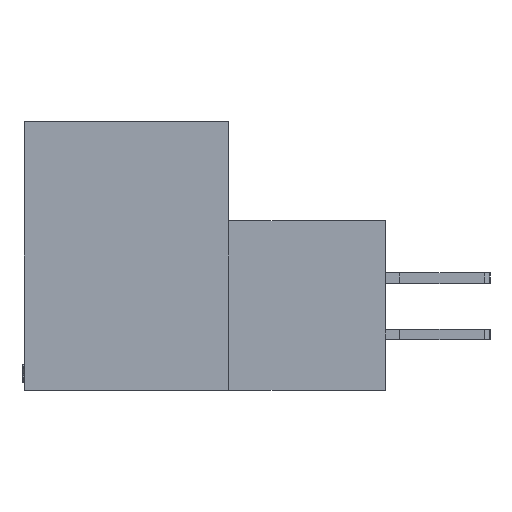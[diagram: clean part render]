
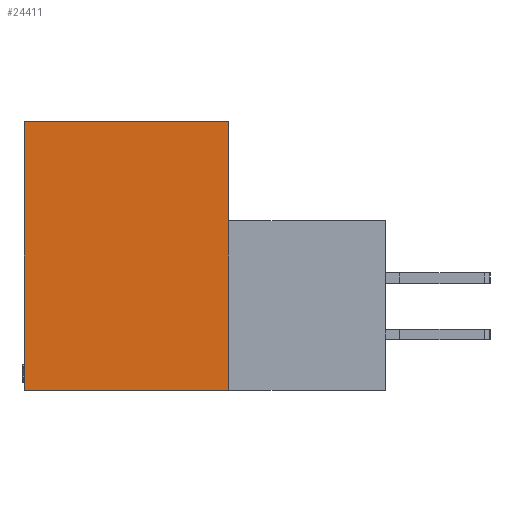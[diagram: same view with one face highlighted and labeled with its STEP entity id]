
A CAD part, left-side view. The second image highlights one B-rep face of the part: STEP entity #24411.
In plain terms, the highlighted planar face has unit normal (-1, 0, 0).
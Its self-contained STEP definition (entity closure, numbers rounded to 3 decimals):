
#324 = EDGE_LOOP ( 'NONE', ( #28597, #47243, #20728, #26605 ) ) ;
#6104 = VERTEX_POINT ( 'NONE', #22603 ) ;
#8108 = DIRECTION ( 'NONE',  ( 0., 1., 0. ) ) ;
#8125 = CARTESIAN_POINT ( 'NONE',  ( 0., 11.506, 0. ) ) ;
#10813 = CARTESIAN_POINT ( 'NONE',  ( 0., 11.506, 0. ) ) ;
#12342 = VERTEX_POINT ( 'NONE', #8125 ) ;
#13488 = DIRECTION ( 'NONE',  ( 0., 0., 1. ) ) ;
#13657 = EDGE_CURVE ( 'NONE', #35111, #43750, #15766, .T. ) ;
#13810 = VECTOR ( 'NONE', #13488, 1000. ) ;
#14408 = EDGE_CURVE ( 'NONE', #43750, #12342, #45364, .T. ) ;
#15766 = LINE ( 'NONE', #31587, #33602 ) ;
#15877 = VECTOR ( 'NONE', #19245, 1000. ) ;
#18761 = PLANE ( 'NONE',  #49935 ) ;
#18810 = CARTESIAN_POINT ( 'NONE',  ( 0., 11.506, -15.088 ) ) ;
#18910 = CARTESIAN_POINT ( 'NONE',  ( 0., 0., 0. ) ) ;
#18948 = CARTESIAN_POINT ( 'NONE',  ( 0., 0., 0. ) ) ;
#19245 = DIRECTION ( 'NONE',  ( 0., 0., -1. ) ) ;
#20728 = ORIENTED_EDGE ( 'NONE', *, *, #32655, .F. ) ;
#22603 = CARTESIAN_POINT ( 'NONE',  ( 0., 0., 0. ) ) ;
#24107 = LINE ( 'NONE', #10813, #32797 ) ;
#24411 = ADVANCED_FACE ( 'NONE', ( #40048 ), #18761, .F. ) ;
#26605 = ORIENTED_EDGE ( 'NONE', *, *, #14408, .F. ) ;
#26664 = DIRECTION ( 'NONE',  ( 0., 0., -1. ) ) ;
#28597 = ORIENTED_EDGE ( 'NONE', *, *, #13657, .F. ) ;
#31587 = CARTESIAN_POINT ( 'NONE',  ( 0., -8.814, -15.088 ) ) ;
#32655 = EDGE_CURVE ( 'NONE', #12342, #6104, #24107, .T. ) ;
#32797 = VECTOR ( 'NONE', #34299, 1000. ) ;
#33602 = VECTOR ( 'NONE', #8108, 1000. ) ;
#34299 = DIRECTION ( 'NONE',  ( 0., -1., 0. ) ) ;
#35111 = VERTEX_POINT ( 'NONE', #45461 ) ;
#38116 = DIRECTION ( 'NONE',  ( 1., 0., 0. ) ) ;
#40048 = FACE_OUTER_BOUND ( 'NONE', #324, .T. ) ;
#43750 = VERTEX_POINT ( 'NONE', #18810 ) ;
#45364 = LINE ( 'NONE', #48604, #13810 ) ;
#45461 = CARTESIAN_POINT ( 'NONE',  ( 0., 0., -15.088 ) ) ;
#47243 = ORIENTED_EDGE ( 'NONE', *, *, #50388, .F. ) ;
#48013 = LINE ( 'NONE', #18910, #15877 ) ;
#48604 = CARTESIAN_POINT ( 'NONE',  ( 0., 11.506, -15.088 ) ) ;
#49935 = AXIS2_PLACEMENT_3D ( 'NONE', #18948, #38116, #26664 ) ;
#50388 = EDGE_CURVE ( 'NONE', #6104, #35111, #48013, .T. ) ;
